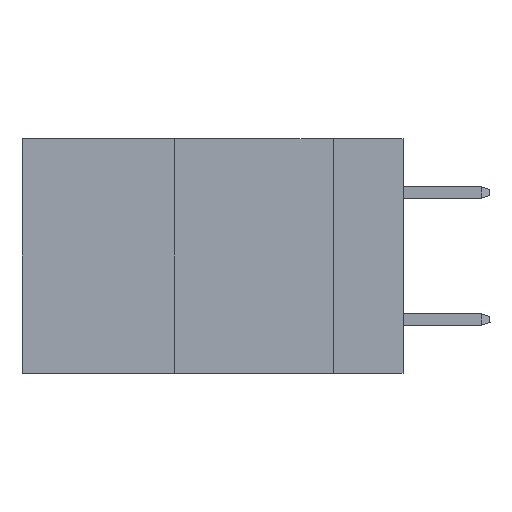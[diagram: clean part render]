
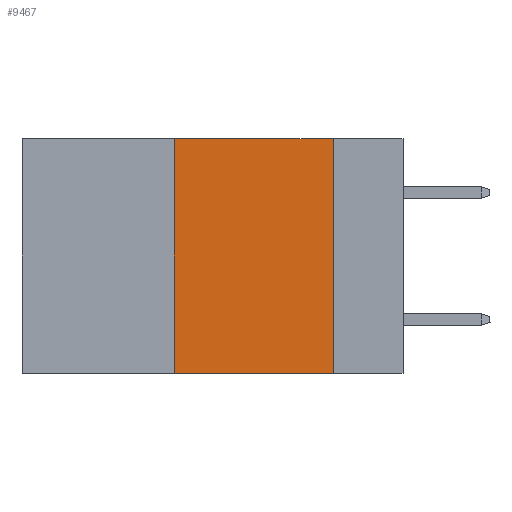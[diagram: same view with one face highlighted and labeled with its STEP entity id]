
A CAD part, left-side view. The second image highlights one B-rep face of the part: STEP entity #9467.
In plain terms, the highlighted planar face has unit normal (-1, 0, 0).
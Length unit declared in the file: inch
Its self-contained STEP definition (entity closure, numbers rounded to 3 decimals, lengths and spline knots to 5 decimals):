
#437 = VERTEX_POINT ( 'NONE', #7789 ) ;
#711 = CARTESIAN_POINT ( 'NONE',  ( 0., 0.6, 0. ) ) ;
#1983 = EDGE_CURVE ( 'NONE', #437, #9738, #9570, .T. ) ;
#3011 = DIRECTION ( 'NONE',  ( 0., -1., 0. ) ) ;
#3317 = AXIS2_PLACEMENT_3D ( 'NONE', #711, #3823, #11988 ) ;
#3554 = ORIENTED_EDGE ( 'NONE', *, *, #1983, .F. ) ;
#3823 = DIRECTION ( 'NONE',  ( 1., 0., 0. ) ) ;
#3888 = VERTEX_POINT ( 'NONE', #9683 ) ;
#4034 = LINE ( 'NONE', #12559, #5927 ) ;
#4246 = DIRECTION ( 'NONE',  ( 0., 0., 1. ) ) ;
#4494 = DIRECTION ( 'NONE',  ( 0., -1., 0. ) ) ;
#5376 = ORIENTED_EDGE ( 'NONE', *, *, #9789, .T. ) ;
#5508 = ORIENTED_EDGE ( 'NONE', *, *, #6882, .F. ) ;
#5907 = VECTOR ( 'NONE', #9753, 39.37008 ) ;
#5927 = VECTOR ( 'NONE', #3011, 39.37008 ) ;
#6330 = CARTESIAN_POINT ( 'NONE',  ( 0., 0.36, 0. ) ) ;
#6378 = LINE ( 'NONE', #8720, #10562 ) ;
#6882 = EDGE_CURVE ( 'NONE', #7254, #3888, #12881, .T. ) ;
#7254 = VERTEX_POINT ( 'NONE', #8224 ) ;
#7552 = CARTESIAN_POINT ( 'NONE',  ( 0., 0.36, 0. ) ) ;
#7789 = CARTESIAN_POINT ( 'NONE',  ( 0., 0.36, -0.37 ) ) ;
#7858 = EDGE_CURVE ( 'NONE', #9738, #7254, #4034, .T. ) ;
#8224 = CARTESIAN_POINT ( 'NONE',  ( 0., 0.11, 0. ) ) ;
#8563 = ORIENTED_EDGE ( 'NONE', *, *, #7858, .F. ) ;
#8720 = CARTESIAN_POINT ( 'NONE',  ( 0., 0.6, -0.37 ) ) ;
#8869 = FACE_OUTER_BOUND ( 'NONE', #12692, .T. ) ;
#9467 = ADVANCED_FACE ( 'NONE', ( #8869 ), #13097, .F. ) ;
#9570 = LINE ( 'NONE', #6330, #11012 ) ;
#9683 = CARTESIAN_POINT ( 'NONE',  ( 0., 0.11, -0.37 ) ) ;
#9738 = VERTEX_POINT ( 'NONE', #7552 ) ;
#9753 = DIRECTION ( 'NONE',  ( 0., 0., -1. ) ) ;
#9789 = EDGE_CURVE ( 'NONE', #437, #3888, #6378, .T. ) ;
#10562 = VECTOR ( 'NONE', #4494, 39.37008 ) ;
#11012 = VECTOR ( 'NONE', #4246, 39.37008 ) ;
#11988 = DIRECTION ( 'NONE',  ( 0., 0., -1. ) ) ;
#12559 = CARTESIAN_POINT ( 'NONE',  ( 0., 0.6, 0. ) ) ;
#12692 = EDGE_LOOP ( 'NONE', ( #5508, #8563, #3554, #5376 ) ) ;
#12822 = CARTESIAN_POINT ( 'NONE',  ( 0., 0.11, 0. ) ) ;
#12881 = LINE ( 'NONE', #12822, #5907 ) ;
#13097 = PLANE ( 'NONE',  #3317 ) ;
